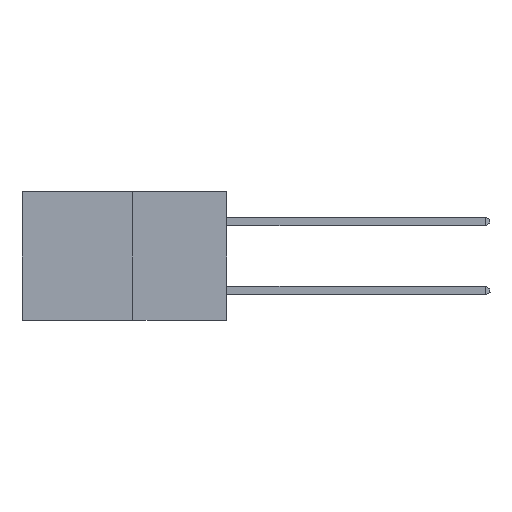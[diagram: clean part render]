
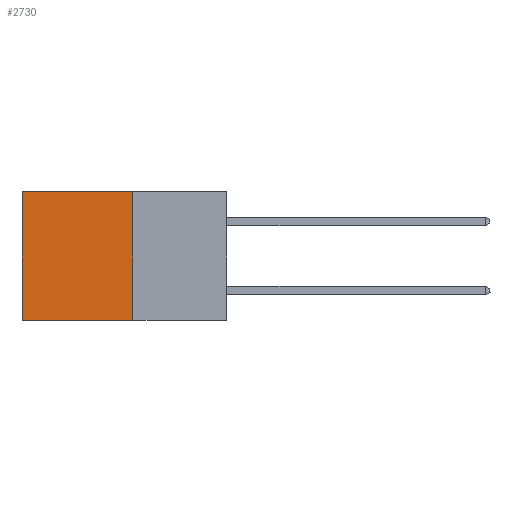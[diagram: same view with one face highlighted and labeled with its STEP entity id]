
A CAD part, left-side view. The second image highlights one B-rep face of the part: STEP entity #2730.
In plain terms, the highlighted planar face has unit normal (-1, 0, 0).
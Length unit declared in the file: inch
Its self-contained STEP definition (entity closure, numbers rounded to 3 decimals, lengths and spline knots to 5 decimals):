
#10 = VERTEX_POINT ( 'NONE', #3492 ) ;
#171 = VERTEX_POINT ( 'NONE', #5364 ) ;
#310 = LINE ( 'NONE', #15929, #18577 ) ;
#1932 = PLANE ( 'NONE',  #3810 ) ;
#2730 = ADVANCED_FACE ( 'NONE', ( #15713 ), #1932, .F. ) ;
#3316 = EDGE_CURVE ( 'NONE', #6715, #10, #17576, .T. ) ;
#3344 = VECTOR ( 'NONE', #12154, 39.37008 ) ;
#3492 = CARTESIAN_POINT ( 'NONE',  ( 0.277, 0.27, -0.37 ) ) ;
#3514 = VECTOR ( 'NONE', #12894, 39.37008 ) ;
#3726 = CARTESIAN_POINT ( 'NONE',  ( 0.277, 0.27, 0. ) ) ;
#3810 = AXIS2_PLACEMENT_3D ( 'NONE', #12513, #16961, #14970 ) ;
#4193 = EDGE_CURVE ( 'NONE', #10, #171, #310, .T. ) ;
#5364 = CARTESIAN_POINT ( 'NONE',  ( 0.277, 0.59, -0.37 ) ) ;
#6330 = EDGE_LOOP ( 'NONE', ( #7733, #8666, #21474, #19785 ) ) ;
#6715 = VERTEX_POINT ( 'NONE', #16423 ) ;
#7151 = LINE ( 'NONE', #3726, #20411 ) ;
#7733 = ORIENTED_EDGE ( 'NONE', *, *, #9905, .T. ) ;
#8666 = ORIENTED_EDGE ( 'NONE', *, *, #4193, .F. ) ;
#8682 = LINE ( 'NONE', #17267, #3344 ) ;
#9844 = DIRECTION ( 'NONE',  ( 0., 1., 0. ) ) ;
#9905 = EDGE_CURVE ( 'NONE', #13805, #171, #8682, .T. ) ;
#12154 = DIRECTION ( 'NONE',  ( 0., 0., -1. ) ) ;
#12513 = CARTESIAN_POINT ( 'NONE',  ( 0.277, 0.27, -0.37 ) ) ;
#12894 = DIRECTION ( 'NONE',  ( 0., 0., -1. ) ) ;
#13514 = CARTESIAN_POINT ( 'NONE',  ( 0.277, 0.27, -0.37 ) ) ;
#13805 = VERTEX_POINT ( 'NONE', #21523 ) ;
#14970 = DIRECTION ( 'NONE',  ( 0., 0., -1. ) ) ;
#15713 = FACE_OUTER_BOUND ( 'NONE', #6330, .T. ) ;
#15929 = CARTESIAN_POINT ( 'NONE',  ( 0.277, 0.27, -0.37 ) ) ;
#16423 = CARTESIAN_POINT ( 'NONE',  ( 0.277, 0.27, 0. ) ) ;
#16961 = DIRECTION ( 'NONE',  ( 1., 0., 0. ) ) ;
#17267 = CARTESIAN_POINT ( 'NONE',  ( 0.277, 0.59, -0.37 ) ) ;
#17319 = EDGE_CURVE ( 'NONE', #6715, #13805, #7151, .T. ) ;
#17576 = LINE ( 'NONE', #13514, #3514 ) ;
#18577 = VECTOR ( 'NONE', #9844, 39.37008 ) ;
#19513 = DIRECTION ( 'NONE',  ( 0., 1., 0. ) ) ;
#19785 = ORIENTED_EDGE ( 'NONE', *, *, #17319, .T. ) ;
#20411 = VECTOR ( 'NONE', #19513, 39.37008 ) ;
#21474 = ORIENTED_EDGE ( 'NONE', *, *, #3316, .F. ) ;
#21523 = CARTESIAN_POINT ( 'NONE',  ( 0.277, 0.59, 0. ) ) ;
